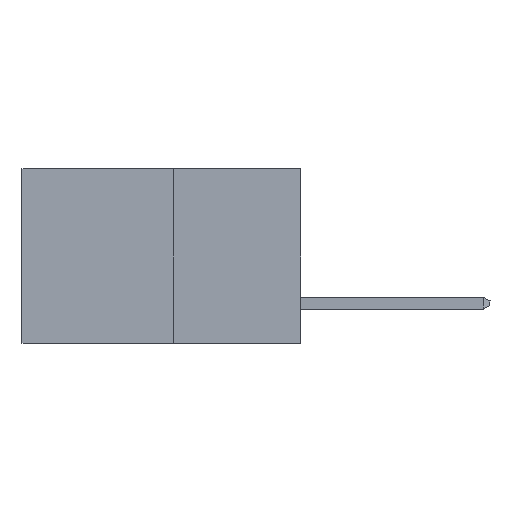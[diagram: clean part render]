
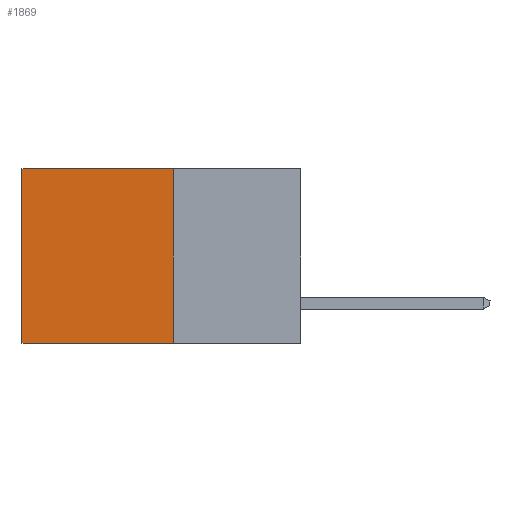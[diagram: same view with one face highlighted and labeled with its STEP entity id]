
A CAD part, left-side view. The second image highlights one B-rep face of the part: STEP entity #1869.
In plain terms, the highlighted planar face has unit normal (-1, 0, 0).
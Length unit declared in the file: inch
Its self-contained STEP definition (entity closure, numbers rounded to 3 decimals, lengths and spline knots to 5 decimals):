
#1110 = CARTESIAN_POINT ( 'NONE',  ( 0.277, 0.27, 0. ) ) ;
#1478 = VERTEX_POINT ( 'NONE', #3955 ) ;
#1858 = CARTESIAN_POINT ( 'NONE',  ( 0.277, 0.27, 0. ) ) ;
#1869 = ADVANCED_FACE ( 'NONE', ( #7171 ), #6316, .F. ) ;
#2521 = VERTEX_POINT ( 'NONE', #9088 ) ;
#2812 = ORIENTED_EDGE ( 'NONE', *, *, #6935, .T. ) ;
#3038 = DIRECTION ( 'NONE',  ( 0., 1., 0. ) ) ;
#3069 = VECTOR ( 'NONE', #3038, 39.37008 ) ;
#3955 = CARTESIAN_POINT ( 'NONE',  ( 0.277, 0.59, 0. ) ) ;
#3971 = DIRECTION ( 'NONE',  ( 0., 0., -1. ) ) ;
#4010 = VECTOR ( 'NONE', #6271, 39.37008 ) ;
#4215 = DIRECTION ( 'NONE',  ( 0., 0., -1. ) ) ;
#4374 = DIRECTION ( 'NONE',  ( 0., 1., 0. ) ) ;
#4411 = EDGE_LOOP ( 'NONE', ( #2812, #9383, #5799, #6845 ) ) ;
#5321 = VERTEX_POINT ( 'NONE', #1110 ) ;
#5364 = AXIS2_PLACEMENT_3D ( 'NONE', #6692, #7937, #4215 ) ;
#5512 = CARTESIAN_POINT ( 'NONE',  ( 0.277, 0.27, -0.37 ) ) ;
#5621 = CARTESIAN_POINT ( 'NONE',  ( 0.277, 0.59, -0.37 ) ) ;
#5799 = ORIENTED_EDGE ( 'NONE', *, *, #8818, .F. ) ;
#6203 = EDGE_CURVE ( 'NONE', #6869, #2521, #9617, .T. ) ;
#6271 = DIRECTION ( 'NONE',  ( 0., 0., -1. ) ) ;
#6284 = LINE ( 'NONE', #5621, #8471 ) ;
#6316 = PLANE ( 'NONE',  #5364 ) ;
#6692 = CARTESIAN_POINT ( 'NONE',  ( 0.277, 0.27, -0.37 ) ) ;
#6845 = ORIENTED_EDGE ( 'NONE', *, *, #7288, .T. ) ;
#6869 = VERTEX_POINT ( 'NONE', #5512 ) ;
#6935 = EDGE_CURVE ( 'NONE', #1478, #2521, #6284, .T. ) ;
#7061 = VECTOR ( 'NONE', #4374, 39.37008 ) ;
#7171 = FACE_OUTER_BOUND ( 'NONE', #4411, .T. ) ;
#7288 = EDGE_CURVE ( 'NONE', #5321, #1478, #7312, .T. ) ;
#7312 = LINE ( 'NONE', #1858, #7061 ) ;
#7937 = DIRECTION ( 'NONE',  ( 1., 0., 0. ) ) ;
#8471 = VECTOR ( 'NONE', #3971, 39.37008 ) ;
#8818 = EDGE_CURVE ( 'NONE', #5321, #6869, #10510, .T. ) ;
#9088 = CARTESIAN_POINT ( 'NONE',  ( 0.277, 0.59, -0.37 ) ) ;
#9383 = ORIENTED_EDGE ( 'NONE', *, *, #6203, .F. ) ;
#9521 = CARTESIAN_POINT ( 'NONE',  ( 0.277, 0.27, -0.37 ) ) ;
#9617 = LINE ( 'NONE', #10370, #3069 ) ;
#10370 = CARTESIAN_POINT ( 'NONE',  ( 0.277, 0.27, -0.37 ) ) ;
#10510 = LINE ( 'NONE', #9521, #4010 ) ;
